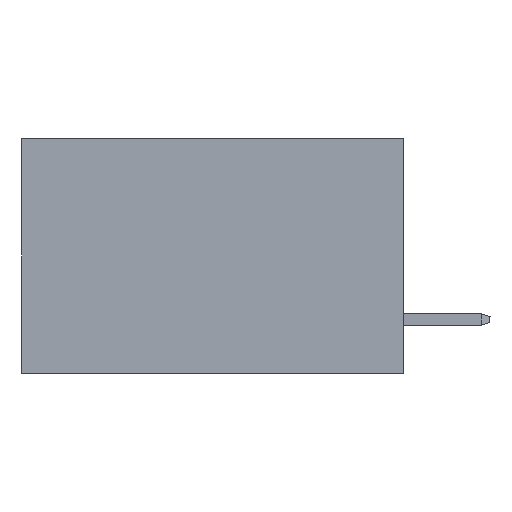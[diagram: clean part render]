
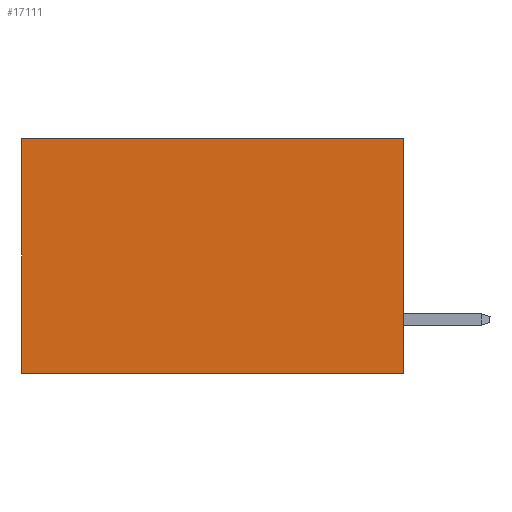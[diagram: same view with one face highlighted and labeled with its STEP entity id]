
A CAD part, left-side view. The second image highlights one B-rep face of the part: STEP entity #17111.
In plain terms, the highlighted planar face has unit normal (-1, 0, 0).
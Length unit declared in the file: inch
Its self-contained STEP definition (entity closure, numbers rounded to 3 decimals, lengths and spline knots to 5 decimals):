
#586 = CARTESIAN_POINT ( 'NONE',  ( 0.2875, 0., 0. ) ) ;
#656 = ORIENTED_EDGE ( 'NONE', *, *, #18143, .F. ) ;
#950 = LINE ( 'NONE', #17907, #3720 ) ;
#1126 = DIRECTION ( 'NONE',  ( 0., 1., 0. ) ) ;
#1221 = CARTESIAN_POINT ( 'NONE',  ( 0.2875, 0., 0. ) ) ;
#2451 = ORIENTED_EDGE ( 'NONE', *, *, #13442, .F. ) ;
#3287 = AXIS2_PLACEMENT_3D ( 'NONE', #1221, #6903, #23997 ) ;
#3720 = VECTOR ( 'NONE', #7131, 39.37008 ) ;
#3741 = CARTESIAN_POINT ( 'NONE',  ( 0.2875, 0.6, -0.37 ) ) ;
#4819 = VERTEX_POINT ( 'NONE', #8883 ) ;
#5731 = LINE ( 'NONE', #23041, #13536 ) ;
#6653 = FACE_OUTER_BOUND ( 'NONE', #9377, .T. ) ;
#6903 = DIRECTION ( 'NONE',  ( 1., 0., 0. ) ) ;
#7131 = DIRECTION ( 'NONE',  ( 0., 1., 0. ) ) ;
#7376 = ORIENTED_EDGE ( 'NONE', *, *, #12820, .T. ) ;
#7822 = LINE ( 'NONE', #18192, #22303 ) ;
#8883 = CARTESIAN_POINT ( 'NONE',  ( 0.2875, 0., -0.37 ) ) ;
#9377 = EDGE_LOOP ( 'NONE', ( #7376, #2451, #656, #17191 ) ) ;
#9532 = VERTEX_POINT ( 'NONE', #21807 ) ;
#12820 = EDGE_CURVE ( 'NONE', #9532, #20272, #5731, .T. ) ;
#12876 = VECTOR ( 'NONE', #24508, 39.37008 ) ;
#13442 = EDGE_CURVE ( 'NONE', #4819, #20272, #7822, .T. ) ;
#13536 = VECTOR ( 'NONE', #21294, 39.37008 ) ;
#17111 = ADVANCED_FACE ( 'NONE', ( #6653 ), #19926, .F. ) ;
#17191 = ORIENTED_EDGE ( 'NONE', *, *, #17328, .T. ) ;
#17328 = EDGE_CURVE ( 'NONE', #17614, #9532, #950, .T. ) ;
#17614 = VERTEX_POINT ( 'NONE', #586 ) ;
#17907 = CARTESIAN_POINT ( 'NONE',  ( 0.2875, 0., 0. ) ) ;
#18143 = EDGE_CURVE ( 'NONE', #17614, #4819, #20781, .T. ) ;
#18192 = CARTESIAN_POINT ( 'NONE',  ( 0.2875, 0., -0.37 ) ) ;
#19926 = PLANE ( 'NONE',  #3287 ) ;
#20272 = VERTEX_POINT ( 'NONE', #3741 ) ;
#20781 = LINE ( 'NONE', #22387, #12876 ) ;
#21294 = DIRECTION ( 'NONE',  ( 0., 0., -1. ) ) ;
#21807 = CARTESIAN_POINT ( 'NONE',  ( 0.2875, 0.6, 0. ) ) ;
#22303 = VECTOR ( 'NONE', #1126, 39.37008 ) ;
#22387 = CARTESIAN_POINT ( 'NONE',  ( 0.2875, 0., 0. ) ) ;
#23041 = CARTESIAN_POINT ( 'NONE',  ( 0.2875, 0.6, 0. ) ) ;
#23997 = DIRECTION ( 'NONE',  ( 0., 0., -1. ) ) ;
#24508 = DIRECTION ( 'NONE',  ( 0., 0., -1. ) ) ;
